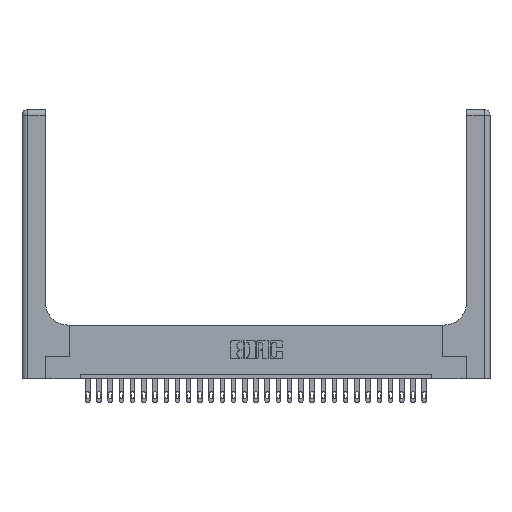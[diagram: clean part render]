
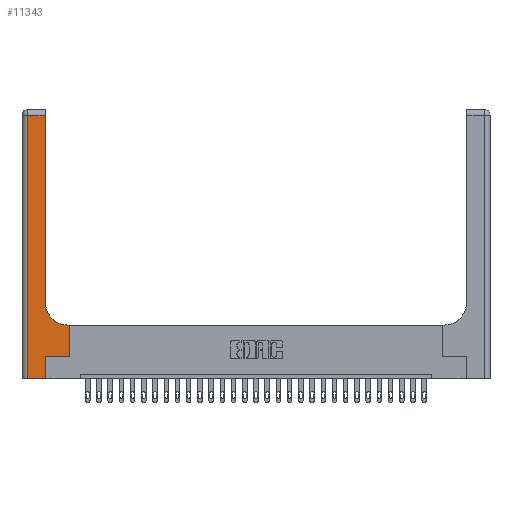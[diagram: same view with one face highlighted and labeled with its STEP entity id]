
A CAD part, top view. The second image highlights one B-rep face of the part: STEP entity #11343.
In plain terms, the highlighted planar face has unit normal (0, 0, 1).
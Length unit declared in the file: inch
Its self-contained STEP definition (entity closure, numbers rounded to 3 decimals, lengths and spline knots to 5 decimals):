
#310 = CARTESIAN_POINT ( 'NONE',  ( 0.265, 0., 0.37 ) ) ;
#1093 = VECTOR ( 'NONE', #3672, 39.37008 ) ;
#1753 = CARTESIAN_POINT ( 'NONE',  ( 0.06, 2.94, 0.37 ) ) ;
#2316 = CARTESIAN_POINT ( 'NONE',  ( 0., 3., 0.37 ) ) ;
#2421 = EDGE_CURVE ( 'NONE', #22674, #17175, #21092, .T. ) ;
#2570 = CARTESIAN_POINT ( 'NONE',  ( 0.528, 0.6, 0.37 ) ) ;
#3428 = VERTEX_POINT ( 'NONE', #18558 ) ;
#3602 = DIRECTION ( 'NONE',  ( 1., 0., 0. ) ) ;
#3672 = DIRECTION ( 'NONE',  ( 0., 1., 0. ) ) ;
#3685 = DIRECTION ( 'NONE',  ( 0., 1., 0. ) ) ;
#3838 = LINE ( 'NONE', #24295, #11136 ) ;
#3881 = DIRECTION ( 'NONE',  ( 0., 1., 0. ) ) ;
#4325 = EDGE_CURVE ( 'NONE', #17175, #19026, #21640, .T. ) ;
#4492 = CARTESIAN_POINT ( 'NONE',  ( 0.265, 0.25, 0.37 ) ) ;
#4877 = CARTESIAN_POINT ( 'NONE',  ( 0.06, 0., 0.37 ) ) ;
#5337 = EDGE_CURVE ( 'NONE', #10624, #3428, #20830, .T. ) ;
#5537 = CARTESIAN_POINT ( 'NONE',  ( 0.528, 0.25, 0.37 ) ) ;
#5601 = EDGE_CURVE ( 'NONE', #19026, #25142, #23525, .T. ) ;
#5758 = CARTESIAN_POINT ( 'NONE',  ( 0.51, 0.85, 0.37 ) ) ;
#5792 = EDGE_CURVE ( 'NONE', #25955, #13860, #15141, .T. ) ;
#6068 = LINE ( 'NONE', #5537, #1093 ) ;
#6978 = VECTOR ( 'NONE', #8771, 39.37008 ) ;
#7039 = AXIS2_PLACEMENT_3D ( 'NONE', #2316, #12412, #10309 ) ;
#7614 = DIRECTION ( 'NONE',  ( 1., 0., 0. ) ) ;
#8101 = DIRECTION ( 'NONE',  ( -1., 0., 0. ) ) ;
#8480 = ORIENTED_EDGE ( 'NONE', *, *, #16340, .T. ) ;
#8771 = DIRECTION ( 'NONE',  ( 1., 0., 0. ) ) ;
#8978 = CARTESIAN_POINT ( 'NONE',  ( 0., 2.94, 0.37 ) ) ;
#9048 = VECTOR ( 'NONE', #11016, 39.37008 ) ;
#9313 = EDGE_LOOP ( 'NONE', ( #22328, #20804, #13449, #24038, #8480, #9356, #18974, #12388, #25209 ) ) ;
#9356 = ORIENTED_EDGE ( 'NONE', *, *, #5792, .T. ) ;
#10177 = PLANE ( 'NONE',  #7039 ) ;
#10309 = DIRECTION ( 'NONE',  ( -1., 0., 0. ) ) ;
#10317 = VERTEX_POINT ( 'NONE', #2570 ) ;
#10624 = VERTEX_POINT ( 'NONE', #18104 ) ;
#10721 = EDGE_CURVE ( 'NONE', #3428, #22674, #13984, .T. ) ;
#11016 = DIRECTION ( 'NONE',  ( 0., -1., 0. ) ) ;
#11136 = VECTOR ( 'NONE', #8101, 39.37008 ) ;
#11343 = ADVANCED_FACE ( 'NONE', ( #22138 ), #10177, .F. ) ;
#11659 = LINE ( 'NONE', #25865, #16696 ) ;
#12388 = ORIENTED_EDGE ( 'NONE', *, *, #14748, .T. ) ;
#12412 = DIRECTION ( 'NONE',  ( 0., 0., -1. ) ) ;
#13449 = ORIENTED_EDGE ( 'NONE', *, *, #4325, .T. ) ;
#13860 = VERTEX_POINT ( 'NONE', #22407 ) ;
#13984 = LINE ( 'NONE', #22100, #14236 ) ;
#14236 = VECTOR ( 'NONE', #3881, 39.37008 ) ;
#14748 = EDGE_CURVE ( 'NONE', #10317, #10624, #3838, .T. ) ;
#15141 = LINE ( 'NONE', #21139, #6978 ) ;
#16340 = EDGE_CURVE ( 'NONE', #25142, #25955, #11659, .T. ) ;
#16696 = VECTOR ( 'NONE', #3685, 39.37008 ) ;
#17175 = VERTEX_POINT ( 'NONE', #1753 ) ;
#17588 = VECTOR ( 'NONE', #3602, 39.37008 ) ;
#18104 = CARTESIAN_POINT ( 'NONE',  ( 0.51, 0.6, 0.37 ) ) ;
#18558 = CARTESIAN_POINT ( 'NONE',  ( 0.26, 0.85, 0.37 ) ) ;
#18974 = ORIENTED_EDGE ( 'NONE', *, *, #23237, .T. ) ;
#19026 = VERTEX_POINT ( 'NONE', #4877 ) ;
#19546 = CARTESIAN_POINT ( 'NONE',  ( 0., 0., 0.37 ) ) ;
#20116 = CARTESIAN_POINT ( 'NONE',  ( 0.26, 2.94, 0.37 ) ) ;
#20804 = ORIENTED_EDGE ( 'NONE', *, *, #2421, .T. ) ;
#20830 = CIRCLE ( 'NONE', #24205, 0.25 ) ;
#21092 = LINE ( 'NONE', #8978, #22960 ) ;
#21139 = CARTESIAN_POINT ( 'NONE',  ( 0.265, 0.25, 0.37 ) ) ;
#21640 = LINE ( 'NONE', #23352, #9048 ) ;
#22100 = CARTESIAN_POINT ( 'NONE',  ( 0.26, 3., 0.37 ) ) ;
#22138 = FACE_OUTER_BOUND ( 'NONE', #9313, .T. ) ;
#22328 = ORIENTED_EDGE ( 'NONE', *, *, #10721, .T. ) ;
#22407 = CARTESIAN_POINT ( 'NONE',  ( 0.528, 0.25, 0.37 ) ) ;
#22674 = VERTEX_POINT ( 'NONE', #20116 ) ;
#22960 = VECTOR ( 'NONE', #25660, 39.37008 ) ;
#23237 = EDGE_CURVE ( 'NONE', #13860, #10317, #6068, .T. ) ;
#23352 = CARTESIAN_POINT ( 'NONE',  ( 0.06, 3., 0.37 ) ) ;
#23525 = LINE ( 'NONE', #19546, #17588 ) ;
#24038 = ORIENTED_EDGE ( 'NONE', *, *, #5601, .T. ) ;
#24205 = AXIS2_PLACEMENT_3D ( 'NONE', #5758, #25800, #7614 ) ;
#24295 = CARTESIAN_POINT ( 'NONE',  ( 0.26, 0.6, 0.37 ) ) ;
#25142 = VERTEX_POINT ( 'NONE', #310 ) ;
#25209 = ORIENTED_EDGE ( 'NONE', *, *, #5337, .T. ) ;
#25660 = DIRECTION ( 'NONE',  ( -1., 0., 0. ) ) ;
#25800 = DIRECTION ( 'NONE',  ( 0., 0., -1. ) ) ;
#25865 = CARTESIAN_POINT ( 'NONE',  ( 0.265, 0., 0.37 ) ) ;
#25955 = VERTEX_POINT ( 'NONE', #4492 ) ;
